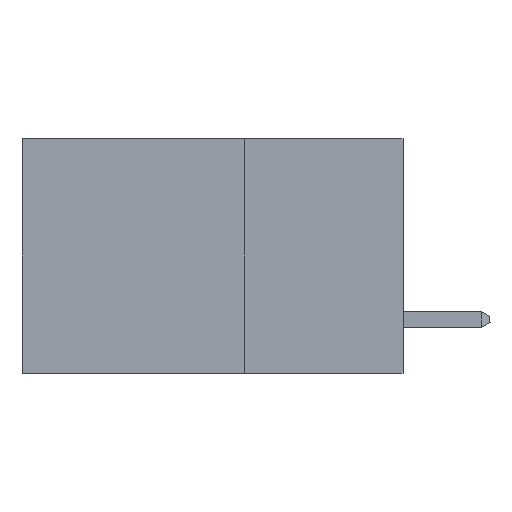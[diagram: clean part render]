
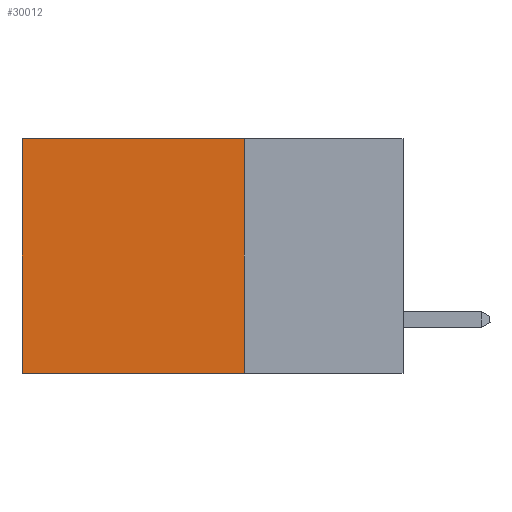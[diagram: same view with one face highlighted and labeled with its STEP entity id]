
A CAD part, left-side view. The second image highlights one B-rep face of the part: STEP entity #30012.
In plain terms, the highlighted planar face has unit normal (-1, 0, 0).
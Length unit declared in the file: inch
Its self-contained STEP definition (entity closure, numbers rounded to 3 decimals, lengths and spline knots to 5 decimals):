
#37 = AXIS2_PLACEMENT_3D ( 'NONE', #5930, #25212, #19787 ) ;
#2661 = DIRECTION ( 'NONE',  ( 0., 1., 0. ) ) ;
#2683 = EDGE_CURVE ( 'NONE', #5413, #20108, #28242, .T. ) ;
#3329 = LINE ( 'NONE', #19176, #19443 ) ;
#5361 = EDGE_LOOP ( 'NONE', ( #11178, #35181, #28035, #25743 ) ) ;
#5413 = VERTEX_POINT ( 'NONE', #25822 ) ;
#5499 = FACE_OUTER_BOUND ( 'NONE', #5361, .T. ) ;
#5930 = CARTESIAN_POINT ( 'NONE',  ( 0.2875, 0.25, 0. ) ) ;
#6034 = PLANE ( 'NONE',  #37 ) ;
#6575 = CARTESIAN_POINT ( 'NONE',  ( 0.2875, 0.6, 0. ) ) ;
#10510 = DIRECTION ( 'NONE',  ( 0., 1., 0. ) ) ;
#11054 = EDGE_CURVE ( 'NONE', #12373, #5413, #3329, .T. ) ;
#11178 = ORIENTED_EDGE ( 'NONE', *, *, #2683, .T. ) ;
#12373 = VERTEX_POINT ( 'NONE', #20753 ) ;
#13153 = LINE ( 'NONE', #17681, #21458 ) ;
#16309 = VECTOR ( 'NONE', #2661, 39.37008 ) ;
#17681 = CARTESIAN_POINT ( 'NONE',  ( 0.2875, 0.25, 0. ) ) ;
#19176 = CARTESIAN_POINT ( 'NONE',  ( 0.2875, 0.25, 0. ) ) ;
#19443 = VECTOR ( 'NONE', #10510, 39.37008 ) ;
#19787 = DIRECTION ( 'NONE',  ( 0., 0., -1. ) ) ;
#20108 = VERTEX_POINT ( 'NONE', #26120 ) ;
#20753 = CARTESIAN_POINT ( 'NONE',  ( 0.2875, 0.25, 0. ) ) ;
#21458 = VECTOR ( 'NONE', #29021, 39.37008 ) ;
#23650 = CARTESIAN_POINT ( 'NONE',  ( 0.2875, 0.25, -0.37 ) ) ;
#25212 = DIRECTION ( 'NONE',  ( 1., 0., 0. ) ) ;
#25743 = ORIENTED_EDGE ( 'NONE', *, *, #11054, .T. ) ;
#25822 = CARTESIAN_POINT ( 'NONE',  ( 0.2875, 0.6, 0. ) ) ;
#26119 = VECTOR ( 'NONE', #28747, 39.37008 ) ;
#26120 = CARTESIAN_POINT ( 'NONE',  ( 0.2875, 0.6, -0.37 ) ) ;
#26248 = LINE ( 'NONE', #27168, #16309 ) ;
#26999 = EDGE_CURVE ( 'NONE', #12373, #27798, #13153, .T. ) ;
#27168 = CARTESIAN_POINT ( 'NONE',  ( 0.2875, 0.25, -0.37 ) ) ;
#27798 = VERTEX_POINT ( 'NONE', #23650 ) ;
#28035 = ORIENTED_EDGE ( 'NONE', *, *, #26999, .F. ) ;
#28242 = LINE ( 'NONE', #6575, #26119 ) ;
#28747 = DIRECTION ( 'NONE',  ( 0., 0., -1. ) ) ;
#29021 = DIRECTION ( 'NONE',  ( 0., 0., -1. ) ) ;
#30012 = ADVANCED_FACE ( 'NONE', ( #5499 ), #6034, .F. ) ;
#31101 = EDGE_CURVE ( 'NONE', #27798, #20108, #26248, .T. ) ;
#35181 = ORIENTED_EDGE ( 'NONE', *, *, #31101, .F. ) ;
